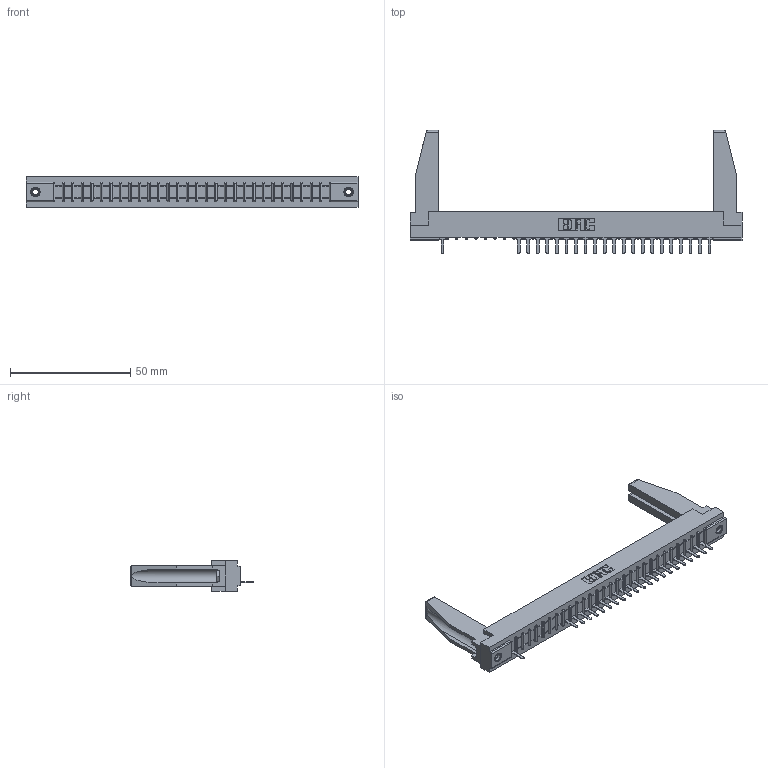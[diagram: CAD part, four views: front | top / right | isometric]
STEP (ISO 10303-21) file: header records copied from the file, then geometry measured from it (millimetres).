
FILE_DESCRIPTION (( 'STEP AP203' ), '1' );
FILE_NAME ('307-029-525-178.STEP', '2018-08-04T17:25:55', ( '' ), ( '' ), 'SwSTEP 2.0', 'SolidWorks 2016', '' );
FILE_SCHEMA (( 'CONFIG_CONTROL_DESIGN' ));
Length unit declared in the file: inch
Products named in the file (5): 307-220-078; 345-250-001_345-250-001-102; 307-029-525-178; 307 Part_.156 Dia Mounting Holes; 307-290-001_525
Assembly tree (27 placements, depth 2):
  307-029-525-178
    307 Part_.156 Dia Mounting Holes
    307-290-001_525  x22
    307-220-078  x2
    345-250-001_345-250-001-102  x2
Bounding box: 137.92 x 51.13 x 12.7 mm (x, y, z)
Volume: 18118.6 mm3; surface area: 17828.9 mm2
Topology: 27 solids, 27 shells, 1650 faces, 4665 edges, 2990 vertices
Faces by surface type: plane 1052, cylinder 522, sphere 60, cone 12, torus 4
Entity records: 28647 total; most frequent: CARTESIAN_POINT 4851, ORIENTED_EDGE 4800, DIRECTION 4674, EDGE_CURVE 2400, VECTOR 1840, LINE 1840, VERTEX_POINT 1552, AXIS2_PLACEMENT_3D 1417
